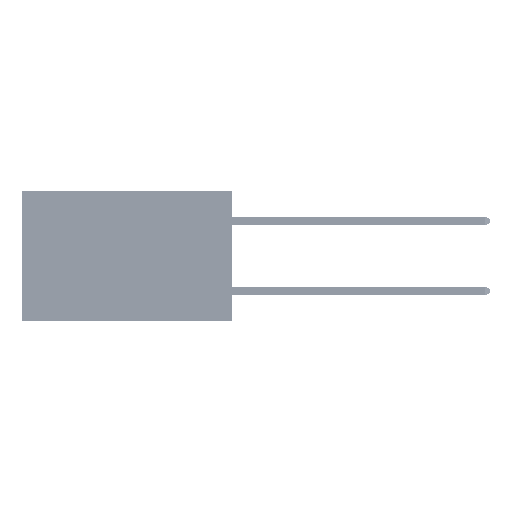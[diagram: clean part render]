
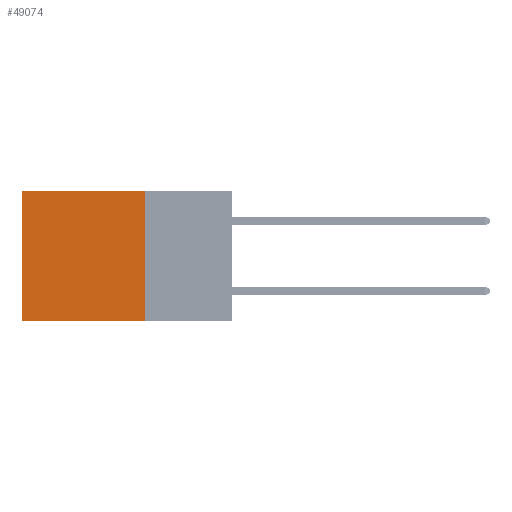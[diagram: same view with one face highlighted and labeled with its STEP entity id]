
A CAD part, left-side view. The second image highlights one B-rep face of the part: STEP entity #49074.
In plain terms, the highlighted planar face has unit normal (-1, 0, 0).
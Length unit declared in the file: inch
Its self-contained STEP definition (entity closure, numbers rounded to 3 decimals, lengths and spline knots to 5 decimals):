
#424 = LINE ( 'NONE', #14295, #32756 ) ;
#1383 = EDGE_CURVE ( 'NONE', #10203, #26248, #424, .T. ) ;
#1391 = CARTESIAN_POINT ( 'NONE',  ( 0.2875, 0.25, 0. ) ) ;
#2911 = CARTESIAN_POINT ( 'NONE',  ( 0.2875, 0.25, 0. ) ) ;
#4371 = LINE ( 'NONE', #27609, #32923 ) ;
#9290 = DIRECTION ( 'NONE',  ( 0., 0., -1. ) ) ;
#9381 = VECTOR ( 'NONE', #20866, 39.37008 ) ;
#10203 = VERTEX_POINT ( 'NONE', #2911 ) ;
#11850 = EDGE_CURVE ( 'NONE', #10203, #40084, #42345, .T. ) ;
#12189 = VECTOR ( 'NONE', #16784, 39.37008 ) ;
#13057 = CARTESIAN_POINT ( 'NONE',  ( 0.2875, 0.25, -0.37 ) ) ;
#13796 = EDGE_LOOP ( 'NONE', ( #37564, #29491, #50808, #27420 ) ) ;
#14295 = CARTESIAN_POINT ( 'NONE',  ( 0.2875, 0.25, 0. ) ) ;
#16784 = DIRECTION ( 'NONE',  ( 0., 1., 0. ) ) ;
#17414 = EDGE_CURVE ( 'NONE', #40084, #32253, #4371, .T. ) ;
#20866 = DIRECTION ( 'NONE',  ( 0., 1., 0. ) ) ;
#25047 = CARTESIAN_POINT ( 'NONE',  ( 0.2875, 0.25, 0. ) ) ;
#25565 = DIRECTION ( 'NONE',  ( 1., 0., 0. ) ) ;
#26248 = VERTEX_POINT ( 'NONE', #36386 ) ;
#27037 = DIRECTION ( 'NONE',  ( 0., 0., -1. ) ) ;
#27420 = ORIENTED_EDGE ( 'NONE', *, *, #11850, .T. ) ;
#27609 = CARTESIAN_POINT ( 'NONE',  ( 0.2875, 0.6, 0. ) ) ;
#29491 = ORIENTED_EDGE ( 'NONE', *, *, #30721, .F. ) ;
#29661 = PLANE ( 'NONE',  #44892 ) ;
#30721 = EDGE_CURVE ( 'NONE', #26248, #32253, #51587, .T. ) ;
#31873 = CARTESIAN_POINT ( 'NONE',  ( 0.2875, 0.6, -0.37 ) ) ;
#32253 = VERTEX_POINT ( 'NONE', #31873 ) ;
#32756 = VECTOR ( 'NONE', #27037, 39.37008 ) ;
#32923 = VECTOR ( 'NONE', #40065, 39.37008 ) ;
#36386 = CARTESIAN_POINT ( 'NONE',  ( 0.2875, 0.25, -0.37 ) ) ;
#37564 = ORIENTED_EDGE ( 'NONE', *, *, #17414, .T. ) ;
#38948 = CARTESIAN_POINT ( 'NONE',  ( 0.2875, 0.6, 0. ) ) ;
#40065 = DIRECTION ( 'NONE',  ( 0., 0., -1. ) ) ;
#40084 = VERTEX_POINT ( 'NONE', #38948 ) ;
#42345 = LINE ( 'NONE', #1391, #9381 ) ;
#44892 = AXIS2_PLACEMENT_3D ( 'NONE', #25047, #25565, #9290 ) ;
#48395 = FACE_OUTER_BOUND ( 'NONE', #13796, .T. ) ;
#49074 = ADVANCED_FACE ( 'NONE', ( #48395 ), #29661, .F. ) ;
#50808 = ORIENTED_EDGE ( 'NONE', *, *, #1383, .F. ) ;
#51587 = LINE ( 'NONE', #13057, #12189 ) ;
